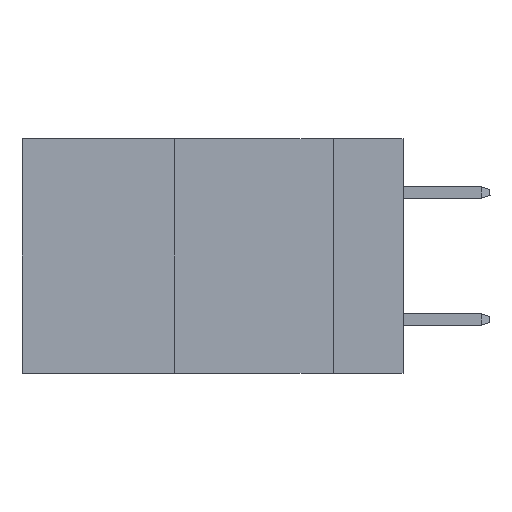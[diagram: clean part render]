
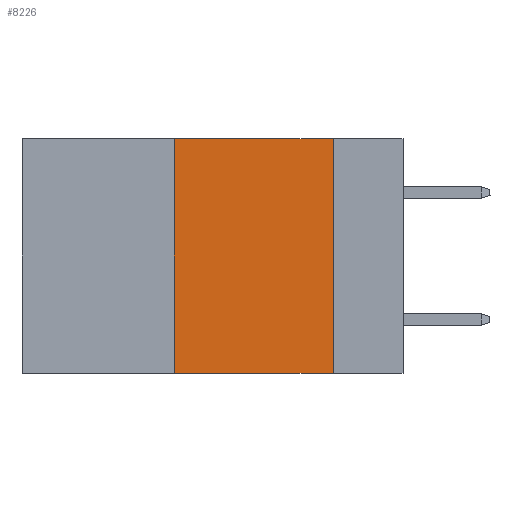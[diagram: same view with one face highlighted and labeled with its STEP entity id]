
A CAD part, left-side view. The second image highlights one B-rep face of the part: STEP entity #8226.
In plain terms, the highlighted planar face has unit normal (-1, 0, 0).
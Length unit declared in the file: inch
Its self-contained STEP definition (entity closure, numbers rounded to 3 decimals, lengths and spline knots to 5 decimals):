
#206 = VERTEX_POINT ( 'NONE', #2854 ) ;
#586 = CARTESIAN_POINT ( 'NONE',  ( 0., 0.6, 0. ) ) ;
#788 = CARTESIAN_POINT ( 'NONE',  ( 0., 0.11, 0. ) ) ;
#1143 = EDGE_CURVE ( 'NONE', #206, #4027, #9702, .T. ) ;
#1220 = CARTESIAN_POINT ( 'NONE',  ( 0., 0.36, 0. ) ) ;
#1458 = VECTOR ( 'NONE', #7792, 39.37008 ) ;
#1506 = LINE ( 'NONE', #788, #1870 ) ;
#1870 = VECTOR ( 'NONE', #9662, 39.37008 ) ;
#2526 = EDGE_LOOP ( 'NONE', ( #6415, #4054, #5292, #2958 ) ) ;
#2552 = CARTESIAN_POINT ( 'NONE',  ( 0., 0.11, 0. ) ) ;
#2780 = EDGE_CURVE ( 'NONE', #4027, #8804, #1506, .T. ) ;
#2854 = CARTESIAN_POINT ( 'NONE',  ( 0., 0.36, 0. ) ) ;
#2958 = ORIENTED_EDGE ( 'NONE', *, *, #8151, .T. ) ;
#3202 = AXIS2_PLACEMENT_3D ( 'NONE', #6292, #3286, #5667 ) ;
#3286 = DIRECTION ( 'NONE',  ( 1., 0., 0. ) ) ;
#3304 = LINE ( 'NONE', #1220, #8190 ) ;
#3803 = VERTEX_POINT ( 'NONE', #9479 ) ;
#4027 = VERTEX_POINT ( 'NONE', #2552 ) ;
#4054 = ORIENTED_EDGE ( 'NONE', *, *, #1143, .F. ) ;
#4189 = VECTOR ( 'NONE', #7573, 39.37008 ) ;
#5010 = CARTESIAN_POINT ( 'NONE',  ( 0., 0.11, -0.37 ) ) ;
#5292 = ORIENTED_EDGE ( 'NONE', *, *, #6427, .F. ) ;
#5667 = DIRECTION ( 'NONE',  ( 0., 0., -1. ) ) ;
#5755 = FACE_OUTER_BOUND ( 'NONE', #2526, .T. ) ;
#6292 = CARTESIAN_POINT ( 'NONE',  ( 0., 0.6, 0. ) ) ;
#6415 = ORIENTED_EDGE ( 'NONE', *, *, #2780, .F. ) ;
#6427 = EDGE_CURVE ( 'NONE', #3803, #206, #3304, .T. ) ;
#7573 = DIRECTION ( 'NONE',  ( 0., -1., 0. ) ) ;
#7746 = LINE ( 'NONE', #9090, #1458 ) ;
#7792 = DIRECTION ( 'NONE',  ( 0., -1., 0. ) ) ;
#8151 = EDGE_CURVE ( 'NONE', #3803, #8804, #7746, .T. ) ;
#8190 = VECTOR ( 'NONE', #9494, 39.37008 ) ;
#8226 = ADVANCED_FACE ( 'NONE', ( #5755 ), #9476, .F. ) ;
#8804 = VERTEX_POINT ( 'NONE', #5010 ) ;
#9090 = CARTESIAN_POINT ( 'NONE',  ( 0., 0.6, -0.37 ) ) ;
#9476 = PLANE ( 'NONE',  #3202 ) ;
#9479 = CARTESIAN_POINT ( 'NONE',  ( 0., 0.36, -0.37 ) ) ;
#9494 = DIRECTION ( 'NONE',  ( 0., 0., 1. ) ) ;
#9662 = DIRECTION ( 'NONE',  ( 0., 0., -1. ) ) ;
#9702 = LINE ( 'NONE', #586, #4189 ) ;
